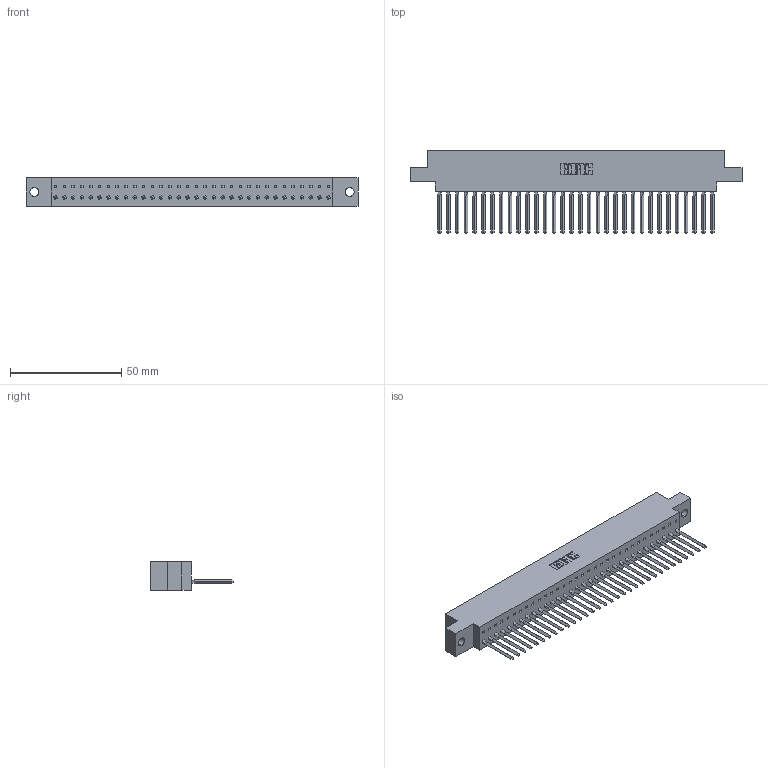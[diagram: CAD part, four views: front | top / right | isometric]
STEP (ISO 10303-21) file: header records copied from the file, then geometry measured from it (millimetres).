
FILE_DESCRIPTION (( 'STEP AP203' ), '1' );
FILE_NAME ('317-032-541-604.STEP', '2020-02-27T21:01:05', ( '' ), ( '' ), 'SwSTEP 2.0', 'SolidWorks 2016', '' );
FILE_SCHEMA (( 'CONFIG_CONTROL_DESIGN' ));
Length unit declared in the file: inch
Products named in the file (3): 317 Part_.156 Dia - TH; 317-032-541-604; 317-290-002_541
Assembly tree (33 placements, depth 2):
  317-032-541-604
    317 Part_.156 Dia - TH
    317-290-002_541  x32
Bounding box: 149.5 x 37.34 x 12.7 mm (x, y, z)
Volume: 23849.3 mm3; surface area: 33185.2 mm2
Topology: 33 solids, 33 shells, 4966 faces, 14163 edges, 9206 vertices
Faces by surface type: plane 4026, cylinder 812, bspline 128
Entity records: 48178 total; most frequent: CARTESIAN_POINT 9201, ORIENTED_EDGE 8486, DIRECTION 6963, EDGE_CURVE 4243, VECTOR 3879, LINE 3879, VERTEX_POINT 2820, AXIS2_PLACEMENT_3D 1542
